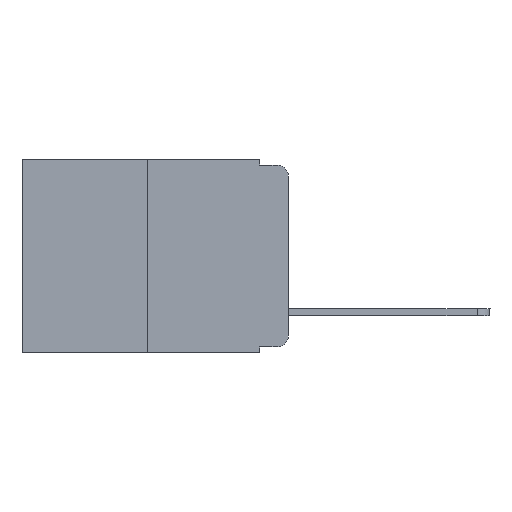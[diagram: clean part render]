
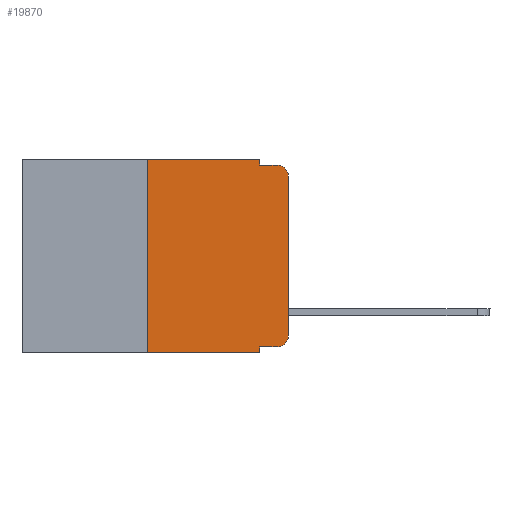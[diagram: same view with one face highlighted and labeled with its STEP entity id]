
A CAD part, left-side view. The second image highlights one B-rep face of the part: STEP entity #19870.
In plain terms, the highlighted planar face has unit normal (-1, 0, 0).
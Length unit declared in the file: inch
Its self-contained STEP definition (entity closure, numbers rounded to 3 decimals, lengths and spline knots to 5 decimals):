
#26 = VERTEX_POINT ( 'NONE', #6182 ) ;
#276 = EDGE_CURVE ( 'NONE', #9127, #11781, #8853, .T. ) ;
#312 = CARTESIAN_POINT ( 'NONE',  ( 0., 0.051, -0.333 ) ) ;
#341 = CARTESIAN_POINT ( 'NONE',  ( 0., 0.25, -0.343 ) ) ;
#458 = LINE ( 'NONE', #3897, #16485 ) ;
#533 = CARTESIAN_POINT ( 'NONE',  ( 0., 0.051, 0. ) ) ;
#1546 = AXIS2_PLACEMENT_3D ( 'NONE', #13685, #10218, #6762 ) ;
#1943 = ORIENTED_EDGE ( 'NONE', *, *, #18205, .F. ) ;
#2038 = PLANE ( 'NONE',  #19158 ) ;
#2067 = CARTESIAN_POINT ( 'NONE',  ( 0., 0., -0.313 ) ) ;
#2713 = LINE ( 'NONE', #7815, #15642 ) ;
#3569 = DIRECTION ( 'NONE',  ( 0., 0., -1. ) ) ;
#3686 = LINE ( 'NONE', #7231, #18621 ) ;
#3744 = CARTESIAN_POINT ( 'NONE',  ( 0., 0.473, -0.343 ) ) ;
#3851 = DIRECTION ( 'NONE',  ( 0., -1., 0. ) ) ;
#3897 = CARTESIAN_POINT ( 'NONE',  ( 0., 0.473, 0. ) ) ;
#3944 = LINE ( 'NONE', #12635, #7140 ) ;
#3949 = ORIENTED_EDGE ( 'NONE', *, *, #6928, .F. ) ;
#4271 = EDGE_CURVE ( 'NONE', #6808, #17506, #13903, .T. ) ;
#4921 = VERTEX_POINT ( 'NONE', #2067 ) ;
#5195 = CARTESIAN_POINT ( 'NONE',  ( 0., 0.02, -0.01 ) ) ;
#5258 = CARTESIAN_POINT ( 'NONE',  ( 0., 0.473, 0. ) ) ;
#5315 = VECTOR ( 'NONE', #18613, 39.37008 ) ;
#5472 = DIRECTION ( 'NONE',  ( 0., 0., -1. ) ) ;
#5571 = EDGE_CURVE ( 'NONE', #13030, #4921, #18990, .T. ) ;
#5671 = EDGE_CURVE ( 'NONE', #9557, #11781, #12565, .T. ) ;
#5733 = CARTESIAN_POINT ( 'NONE',  ( 0., 0.02, -0.333 ) ) ;
#6025 = ORIENTED_EDGE ( 'NONE', *, *, #15375, .T. ) ;
#6182 = CARTESIAN_POINT ( 'NONE',  ( 0., 0., -0.03 ) ) ;
#6205 = VECTOR ( 'NONE', #10986, 39.37008 ) ;
#6332 = ORIENTED_EDGE ( 'NONE', *, *, #5671, .F. ) ;
#6759 = CARTESIAN_POINT ( 'NONE',  ( 0., 0.051, 0. ) ) ;
#6762 = DIRECTION ( 'NONE',  ( 0., 0., -1. ) ) ;
#6793 = CARTESIAN_POINT ( 'NONE',  ( 0., 0.051, 0. ) ) ;
#6808 = VERTEX_POINT ( 'NONE', #6793 ) ;
#6928 = EDGE_CURVE ( 'NONE', #8857, #6808, #458, .T. ) ;
#6963 = EDGE_CURVE ( 'NONE', #9557, #13030, #3686, .T. ) ;
#7140 = VECTOR ( 'NONE', #17436, 39.37008 ) ;
#7231 = CARTESIAN_POINT ( 'NONE',  ( 0., 0.051, -0.333 ) ) ;
#7579 = CARTESIAN_POINT ( 'NONE',  ( 0., 0.25, 0. ) ) ;
#7815 = CARTESIAN_POINT ( 'NONE',  ( 0., 0.051, -0.01 ) ) ;
#8643 = ORIENTED_EDGE ( 'NONE', *, *, #16659, .F. ) ;
#8853 = LINE ( 'NONE', #3744, #15997 ) ;
#8857 = VERTEX_POINT ( 'NONE', #7579 ) ;
#9127 = VERTEX_POINT ( 'NONE', #341 ) ;
#9231 = DIRECTION ( 'NONE',  ( 0., -1., 0. ) ) ;
#9557 = VERTEX_POINT ( 'NONE', #312 ) ;
#10218 = DIRECTION ( 'NONE',  ( -1., 0., 0. ) ) ;
#10489 = DIRECTION ( 'NONE',  ( 1., 0., 0. ) ) ;
#10986 = DIRECTION ( 'NONE',  ( 0., 0., -1. ) ) ;
#11331 = CARTESIAN_POINT ( 'NONE',  ( 0., 0.051, -0.01 ) ) ;
#11452 = VECTOR ( 'NONE', #17252, 39.37008 ) ;
#11781 = VERTEX_POINT ( 'NONE', #19220 ) ;
#12565 = LINE ( 'NONE', #533, #6205 ) ;
#12635 = CARTESIAN_POINT ( 'NONE',  ( 0., 0.25, 0. ) ) ;
#12952 = DIRECTION ( 'NONE',  ( 0., -1., 0. ) ) ;
#13030 = VERTEX_POINT ( 'NONE', #5733 ) ;
#13685 = CARTESIAN_POINT ( 'NONE',  ( 0., 0.02, -0.313 ) ) ;
#13903 = LINE ( 'NONE', #6759, #11452 ) ;
#14087 = ORIENTED_EDGE ( 'NONE', *, *, #6963, .T. ) ;
#15294 = ORIENTED_EDGE ( 'NONE', *, *, #18459, .T. ) ;
#15375 = EDGE_CURVE ( 'NONE', #4921, #26, #21966, .T. ) ;
#15642 = VECTOR ( 'NONE', #12952, 39.37008 ) ;
#15886 = VERTEX_POINT ( 'NONE', #5195 ) ;
#15997 = VECTOR ( 'NONE', #3851, 39.37008 ) ;
#16077 = CIRCLE ( 'NONE', #18922, 0.02 ) ;
#16485 = VECTOR ( 'NONE', #9231, 39.37008 ) ;
#16659 = EDGE_CURVE ( 'NONE', #17506, #15886, #2713, .T. ) ;
#16718 = CARTESIAN_POINT ( 'NONE',  ( 0., 0., 0. ) ) ;
#17252 = DIRECTION ( 'NONE',  ( 0., 0., -1. ) ) ;
#17282 = DIRECTION ( 'NONE',  ( 0., -1., 0. ) ) ;
#17436 = DIRECTION ( 'NONE',  ( 0., 0., 1. ) ) ;
#17506 = VERTEX_POINT ( 'NONE', #11331 ) ;
#18205 = EDGE_CURVE ( 'NONE', #9127, #8857, #3944, .T. ) ;
#18459 = EDGE_CURVE ( 'NONE', #26, #15886, #16077, .T. ) ;
#18613 = DIRECTION ( 'NONE',  ( 0., 0., 1. ) ) ;
#18621 = VECTOR ( 'NONE', #17282, 39.37008 ) ;
#18652 = FACE_OUTER_BOUND ( 'NONE', #19978, .T. ) ;
#18844 = CARTESIAN_POINT ( 'NONE',  ( 0., 0.02, -0.03 ) ) ;
#18922 = AXIS2_PLACEMENT_3D ( 'NONE', #18844, #19287, #3569 ) ;
#18990 = CIRCLE ( 'NONE', #1546, 0.02 ) ;
#19158 = AXIS2_PLACEMENT_3D ( 'NONE', #5258, #10489, #5472 ) ;
#19220 = CARTESIAN_POINT ( 'NONE',  ( 0., 0.051, -0.343 ) ) ;
#19287 = DIRECTION ( 'NONE',  ( -1., 0., 0. ) ) ;
#19509 = ORIENTED_EDGE ( 'NONE', *, *, #276, .T. ) ;
#19870 = ADVANCED_FACE ( 'NONE', ( #18652 ), #2038, .F. ) ;
#19978 = EDGE_LOOP ( 'NONE', ( #6025, #15294, #8643, #20608, #3949, #1943, #19509, #6332, #14087, #21321 ) ) ;
#20608 = ORIENTED_EDGE ( 'NONE', *, *, #4271, .F. ) ;
#21321 = ORIENTED_EDGE ( 'NONE', *, *, #5571, .T. ) ;
#21966 = LINE ( 'NONE', #16718, #5315 ) ;
